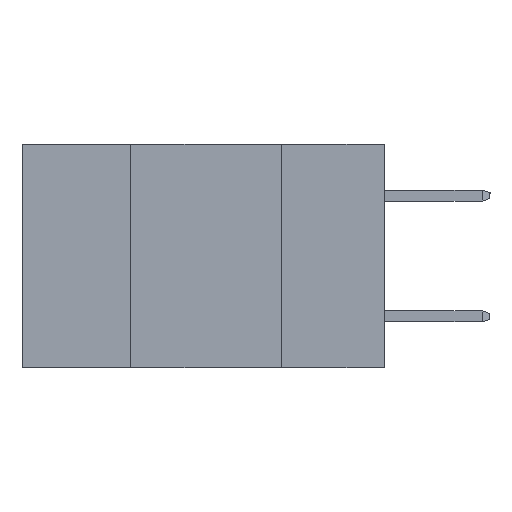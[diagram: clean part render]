
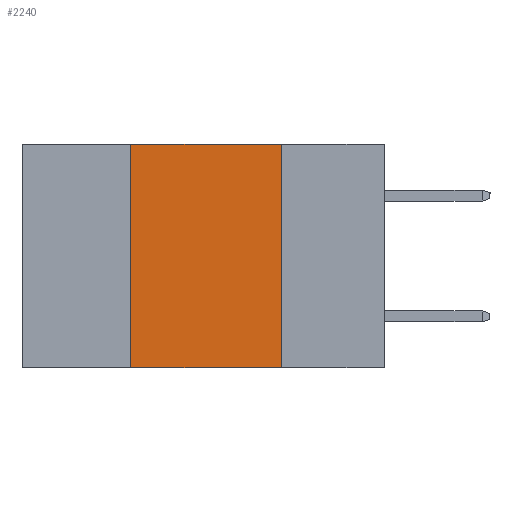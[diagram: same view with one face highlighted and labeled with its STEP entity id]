
A CAD part, left-side view. The second image highlights one B-rep face of the part: STEP entity #2240.
In plain terms, the highlighted planar face has unit normal (-1, 0, 0).
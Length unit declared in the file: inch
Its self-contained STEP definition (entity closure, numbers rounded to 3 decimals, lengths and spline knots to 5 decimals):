
#927 = VERTEX_POINT ( 'NONE', #10207 ) ;
#1755 = DIRECTION ( 'NONE',  ( 0., 0., 1. ) ) ;
#1761 = LINE ( 'NONE', #8751, #7344 ) ;
#2240 = ADVANCED_FACE ( 'NONE', ( #15010 ), #21993, .F. ) ;
#2738 = ORIENTED_EDGE ( 'NONE', *, *, #6391, .F. ) ;
#2864 = DIRECTION ( 'NONE',  ( 0., -1., 0. ) ) ;
#3899 = DIRECTION ( 'NONE',  ( 0., 0., -1. ) ) ;
#5426 = CARTESIAN_POINT ( 'NONE',  ( 0., 0.42, -0.37 ) ) ;
#5962 = LINE ( 'NONE', #18237, #10999 ) ;
#6391 = EDGE_CURVE ( 'NONE', #16126, #927, #5962, .T. ) ;
#6624 = CARTESIAN_POINT ( 'NONE',  ( 0., 0.42, -0.37 ) ) ;
#7065 = EDGE_CURVE ( 'NONE', #18896, #17029, #1761, .T. ) ;
#7344 = VECTOR ( 'NONE', #14713, 39.37008 ) ;
#7920 = AXIS2_PLACEMENT_3D ( 'NONE', #13271, #20280, #11551 ) ;
#7935 = ORIENTED_EDGE ( 'NONE', *, *, #16925, .F. ) ;
#8751 = CARTESIAN_POINT ( 'NONE',  ( 0., 0.6, -0.37 ) ) ;
#10207 = CARTESIAN_POINT ( 'NONE',  ( 0., 0.17, 0. ) ) ;
#10999 = VECTOR ( 'NONE', #2864, 39.37008 ) ;
#11551 = DIRECTION ( 'NONE',  ( 0., 0., -1. ) ) ;
#12026 = VECTOR ( 'NONE', #3899, 39.37008 ) ;
#12172 = LINE ( 'NONE', #5426, #14787 ) ;
#12464 = EDGE_LOOP ( 'NONE', ( #7935, #2738, #14539, #14687 ) ) ;
#13271 = CARTESIAN_POINT ( 'NONE',  ( 0., 0.6, 0. ) ) ;
#14539 = ORIENTED_EDGE ( 'NONE', *, *, #19994, .F. ) ;
#14687 = ORIENTED_EDGE ( 'NONE', *, *, #7065, .T. ) ;
#14713 = DIRECTION ( 'NONE',  ( 0., -1., 0. ) ) ;
#14787 = VECTOR ( 'NONE', #1755, 39.37008 ) ;
#15010 = FACE_OUTER_BOUND ( 'NONE', #12464, .T. ) ;
#15498 = CARTESIAN_POINT ( 'NONE',  ( 0., 0.42, 0. ) ) ;
#16126 = VERTEX_POINT ( 'NONE', #15498 ) ;
#16396 = CARTESIAN_POINT ( 'NONE',  ( 0., 0.17, -0.37 ) ) ;
#16925 = EDGE_CURVE ( 'NONE', #927, #17029, #17884, .T. ) ;
#17029 = VERTEX_POINT ( 'NONE', #16396 ) ;
#17884 = LINE ( 'NONE', #21772, #12026 ) ;
#18237 = CARTESIAN_POINT ( 'NONE',  ( 0., 0.6, 0. ) ) ;
#18896 = VERTEX_POINT ( 'NONE', #6624 ) ;
#19994 = EDGE_CURVE ( 'NONE', #18896, #16126, #12172, .T. ) ;
#20280 = DIRECTION ( 'NONE',  ( 1., 0., 0. ) ) ;
#21772 = CARTESIAN_POINT ( 'NONE',  ( 0., 0.17, -0.37 ) ) ;
#21993 = PLANE ( 'NONE',  #7920 ) ;
